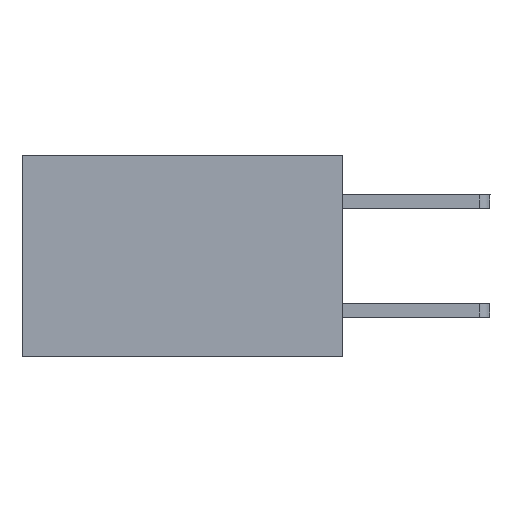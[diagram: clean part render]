
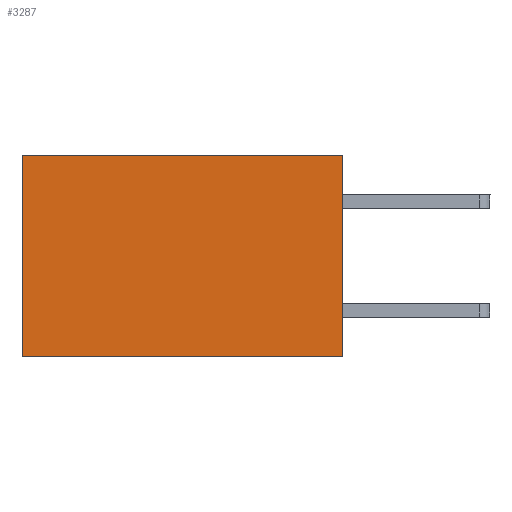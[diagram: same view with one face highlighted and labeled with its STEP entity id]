
A CAD part, left-side view. The second image highlights one B-rep face of the part: STEP entity #3287.
In plain terms, the highlighted planar face has unit normal (-1, 0, 0).
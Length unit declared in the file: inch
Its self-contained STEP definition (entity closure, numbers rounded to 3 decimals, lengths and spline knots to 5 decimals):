
#63 = CARTESIAN_POINT ( 'NONE',  ( 0.277, 0., 0. ) ) ;
#160 = VECTOR ( 'NONE', #2636, 39.37008 ) ;
#1281 = VERTEX_POINT ( 'NONE', #6987 ) ;
#1735 = DIRECTION ( 'NONE',  ( 0., 0., -1. ) ) ;
#2100 = EDGE_CURVE ( 'NONE', #1281, #4832, #11968, .T. ) ;
#2289 = CARTESIAN_POINT ( 'NONE',  ( 0.277, 0.59, 0. ) ) ;
#2591 = LINE ( 'NONE', #2837, #7971 ) ;
#2636 = DIRECTION ( 'NONE',  ( 0., 0., -1. ) ) ;
#2737 = VECTOR ( 'NONE', #3601, 39.37008 ) ;
#2837 = CARTESIAN_POINT ( 'NONE',  ( 0.277, 0.59, -0.37 ) ) ;
#3205 = EDGE_CURVE ( 'NONE', #9109, #4832, #2591, .T. ) ;
#3287 = ADVANCED_FACE ( 'NONE', ( #8436 ), #4708, .F. ) ;
#3338 = ORIENTED_EDGE ( 'NONE', *, *, #5492, .T. ) ;
#3601 = DIRECTION ( 'NONE',  ( 0., 1., 0. ) ) ;
#3658 = DIRECTION ( 'NONE',  ( 1., 0., 0. ) ) ;
#3708 = CARTESIAN_POINT ( 'NONE',  ( 0.277, 0., -0.37 ) ) ;
#3754 = EDGE_CURVE ( 'NONE', #7529, #1281, #11067, .T. ) ;
#4708 = PLANE ( 'NONE',  #8540 ) ;
#4832 = VERTEX_POINT ( 'NONE', #10813 ) ;
#5308 = ORIENTED_EDGE ( 'NONE', *, *, #3754, .F. ) ;
#5492 = EDGE_CURVE ( 'NONE', #7529, #9109, #8039, .T. ) ;
#6194 = CARTESIAN_POINT ( 'NONE',  ( 0.277, 0., 0. ) ) ;
#6987 = CARTESIAN_POINT ( 'NONE',  ( 0.277, 0., -0.37 ) ) ;
#7529 = VERTEX_POINT ( 'NONE', #63 ) ;
#7971 = VECTOR ( 'NONE', #1735, 39.37008 ) ;
#8039 = LINE ( 'NONE', #6194, #9143 ) ;
#8276 = DIRECTION ( 'NONE',  ( 0., 1., 0. ) ) ;
#8308 = DIRECTION ( 'NONE',  ( 0., 0., -1. ) ) ;
#8370 = CARTESIAN_POINT ( 'NONE',  ( 0.277, 0., -0.37 ) ) ;
#8436 = FACE_OUTER_BOUND ( 'NONE', #10953, .T. ) ;
#8540 = AXIS2_PLACEMENT_3D ( 'NONE', #8370, #3658, #8308 ) ;
#9109 = VERTEX_POINT ( 'NONE', #2289 ) ;
#9143 = VECTOR ( 'NONE', #8276, 39.37008 ) ;
#10813 = CARTESIAN_POINT ( 'NONE',  ( 0.277, 0.59, -0.37 ) ) ;
#10953 = EDGE_LOOP ( 'NONE', ( #11662, #11511, #5308, #3338 ) ) ;
#11067 = LINE ( 'NONE', #3708, #160 ) ;
#11511 = ORIENTED_EDGE ( 'NONE', *, *, #2100, .F. ) ;
#11662 = ORIENTED_EDGE ( 'NONE', *, *, #3205, .T. ) ;
#11968 = LINE ( 'NONE', #12026, #2737 ) ;
#12026 = CARTESIAN_POINT ( 'NONE',  ( 0.277, 0., -0.37 ) ) ;
